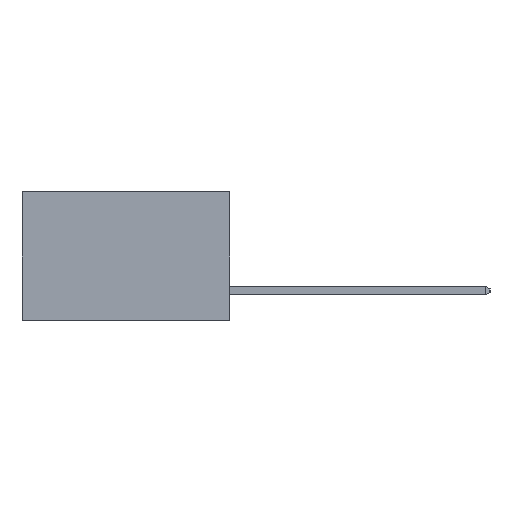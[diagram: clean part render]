
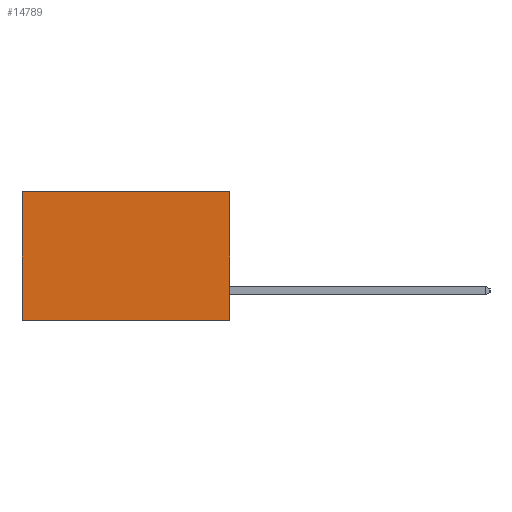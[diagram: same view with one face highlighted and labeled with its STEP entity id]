
A CAD part, left-side view. The second image highlights one B-rep face of the part: STEP entity #14789.
In plain terms, the highlighted planar face has unit normal (-1, 0, 0).
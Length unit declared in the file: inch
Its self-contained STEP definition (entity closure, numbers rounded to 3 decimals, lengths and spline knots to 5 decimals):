
#1601 = EDGE_LOOP ( 'NONE', ( #1969, #15716, #21180, #3909 ) ) ;
#1780 = EDGE_CURVE ( 'NONE', #2392, #16788, #13427, .T. ) ;
#1969 = ORIENTED_EDGE ( 'NONE', *, *, #1780, .T. ) ;
#2369 = LINE ( 'NONE', #17961, #20539 ) ;
#2392 = VERTEX_POINT ( 'NONE', #20377 ) ;
#3021 = DIRECTION ( 'NONE',  ( 0., 0., -1. ) ) ;
#3024 = DIRECTION ( 'NONE',  ( 1., 0., 0. ) ) ;
#3049 = CARTESIAN_POINT ( 'NONE',  ( 0.2615, 0., -0.37 ) ) ;
#3136 = PLANE ( 'NONE',  #20642 ) ;
#3909 = ORIENTED_EDGE ( 'NONE', *, *, #18186, .T. ) ;
#4300 = EDGE_CURVE ( 'NONE', #5866, #14576, #22543, .T. ) ;
#4479 = VECTOR ( 'NONE', #19132, 39.37008 ) ;
#5823 = DIRECTION ( 'NONE',  ( 0., 0., -1. ) ) ;
#5866 = VERTEX_POINT ( 'NONE', #20992 ) ;
#6147 = CARTESIAN_POINT ( 'NONE',  ( 0.2615, 0., -0.37 ) ) ;
#6480 = CARTESIAN_POINT ( 'NONE',  ( 0.2615, 0., -0.37 ) ) ;
#8537 = CARTESIAN_POINT ( 'NONE',  ( 0.2615, 0.6, -0.37 ) ) ;
#8920 = DIRECTION ( 'NONE',  ( 0., 0., -1. ) ) ;
#9577 = VECTOR ( 'NONE', #5823, 39.37008 ) ;
#13268 = CARTESIAN_POINT ( 'NONE',  ( 0.2615, 0.6, -0.37 ) ) ;
#13427 = LINE ( 'NONE', #8537, #17528 ) ;
#14576 = VERTEX_POINT ( 'NONE', #6480 ) ;
#14789 = ADVANCED_FACE ( 'NONE', ( #22032 ), #3136, .F. ) ;
#15305 = EDGE_CURVE ( 'NONE', #14576, #16788, #2369, .T. ) ;
#15716 = ORIENTED_EDGE ( 'NONE', *, *, #15305, .F. ) ;
#16788 = VERTEX_POINT ( 'NONE', #13268 ) ;
#17528 = VECTOR ( 'NONE', #8920, 39.37008 ) ;
#17961 = CARTESIAN_POINT ( 'NONE',  ( 0.2615, 0., -0.37 ) ) ;
#17998 = DIRECTION ( 'NONE',  ( 0., 1., 0. ) ) ;
#18186 = EDGE_CURVE ( 'NONE', #5866, #2392, #18775, .T. ) ;
#18775 = LINE ( 'NONE', #19365, #4479 ) ;
#19132 = DIRECTION ( 'NONE',  ( 0., 1., 0. ) ) ;
#19365 = CARTESIAN_POINT ( 'NONE',  ( 0.2615, 0., 0. ) ) ;
#20377 = CARTESIAN_POINT ( 'NONE',  ( 0.2615, 0.6, 0. ) ) ;
#20539 = VECTOR ( 'NONE', #17998, 39.37008 ) ;
#20642 = AXIS2_PLACEMENT_3D ( 'NONE', #3049, #3024, #3021 ) ;
#20992 = CARTESIAN_POINT ( 'NONE',  ( 0.2615, 0., 0. ) ) ;
#21180 = ORIENTED_EDGE ( 'NONE', *, *, #4300, .F. ) ;
#22032 = FACE_OUTER_BOUND ( 'NONE', #1601, .T. ) ;
#22543 = LINE ( 'NONE', #6147, #9577 ) ;
